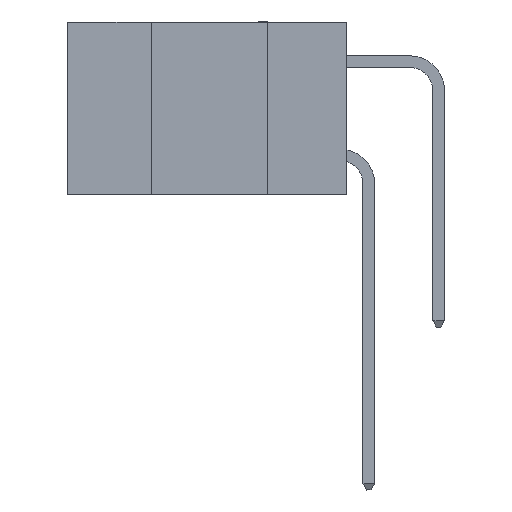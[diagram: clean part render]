
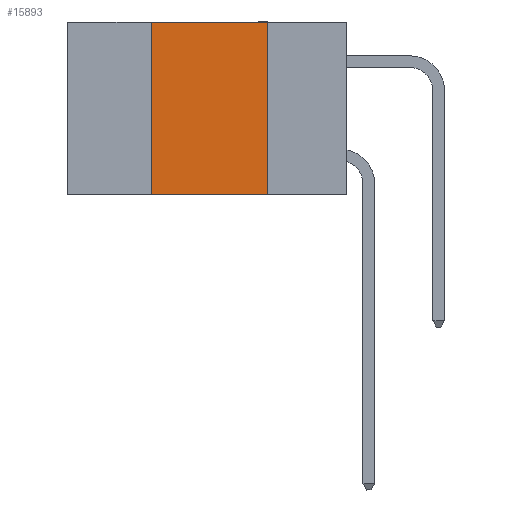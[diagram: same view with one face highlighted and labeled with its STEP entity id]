
A CAD part, left-side view. The second image highlights one B-rep face of the part: STEP entity #15893.
In plain terms, the highlighted planar face has unit normal (-1, 0, 0).
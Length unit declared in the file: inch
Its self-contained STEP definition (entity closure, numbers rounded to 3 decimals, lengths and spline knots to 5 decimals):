
#750 = DIRECTION ( 'NONE',  ( 0., 0., 1. ) ) ;
#959 = CARTESIAN_POINT ( 'NONE',  ( 0., 0.42, -0.37 ) ) ;
#1718 = EDGE_CURVE ( 'NONE', #34587, #13368, #12573, .T. ) ;
#2659 = ORIENTED_EDGE ( 'NONE', *, *, #25937, .F. ) ;
#3508 = CARTESIAN_POINT ( 'NONE',  ( 0., 0.17, -0.37 ) ) ;
#3597 = DIRECTION ( 'NONE',  ( 0., -1., 0. ) ) ;
#5549 = PLANE ( 'NONE',  #23529 ) ;
#7047 = CARTESIAN_POINT ( 'NONE',  ( 0., 0.17, 0. ) ) ;
#7544 = CARTESIAN_POINT ( 'NONE',  ( 0., 0.6, 0. ) ) ;
#8342 = DIRECTION ( 'NONE',  ( 1., 0., 0. ) ) ;
#12573 = LINE ( 'NONE', #20277, #33843 ) ;
#13353 = LINE ( 'NONE', #7544, #21635 ) ;
#13368 = VERTEX_POINT ( 'NONE', #3508 ) ;
#14957 = ORIENTED_EDGE ( 'NONE', *, *, #31328, .F. ) ;
#15893 = ADVANCED_FACE ( 'NONE', ( #24426 ), #5549, .F. ) ;
#15953 = EDGE_LOOP ( 'NONE', ( #2659, #14957, #34130, #21991 ) ) ;
#16628 = EDGE_CURVE ( 'NONE', #34587, #33032, #29564, .T. ) ;
#16798 = LINE ( 'NONE', #23496, #30723 ) ;
#20139 = CARTESIAN_POINT ( 'NONE',  ( 0., 0.42, 0. ) ) ;
#20277 = CARTESIAN_POINT ( 'NONE',  ( 0., 0.6, -0.37 ) ) ;
#21587 = VERTEX_POINT ( 'NONE', #7047 ) ;
#21635 = VECTOR ( 'NONE', #27052, 39.37008 ) ;
#21991 = ORIENTED_EDGE ( 'NONE', *, *, #1718, .T. ) ;
#22172 = VECTOR ( 'NONE', #750, 39.37008 ) ;
#22932 = CARTESIAN_POINT ( 'NONE',  ( 0., 0.42, 0. ) ) ;
#23496 = CARTESIAN_POINT ( 'NONE',  ( 0., 0.17, 0. ) ) ;
#23529 = AXIS2_PLACEMENT_3D ( 'NONE', #30491, #8342, #27844 ) ;
#24426 = FACE_OUTER_BOUND ( 'NONE', #15953, .T. ) ;
#25937 = EDGE_CURVE ( 'NONE', #21587, #13368, #16798, .T. ) ;
#26320 = DIRECTION ( 'NONE',  ( 0., 0., -1. ) ) ;
#27052 = DIRECTION ( 'NONE',  ( 0., -1., 0. ) ) ;
#27844 = DIRECTION ( 'NONE',  ( 0., 0., -1. ) ) ;
#29564 = LINE ( 'NONE', #20139, #22172 ) ;
#30491 = CARTESIAN_POINT ( 'NONE',  ( 0., 0.6, 0. ) ) ;
#30723 = VECTOR ( 'NONE', #26320, 39.37008 ) ;
#31328 = EDGE_CURVE ( 'NONE', #33032, #21587, #13353, .T. ) ;
#33032 = VERTEX_POINT ( 'NONE', #22932 ) ;
#33843 = VECTOR ( 'NONE', #3597, 39.37008 ) ;
#34130 = ORIENTED_EDGE ( 'NONE', *, *, #16628, .F. ) ;
#34587 = VERTEX_POINT ( 'NONE', #959 ) ;
